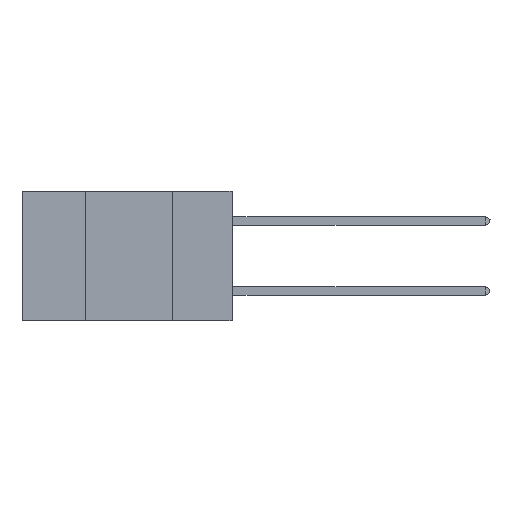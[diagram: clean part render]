
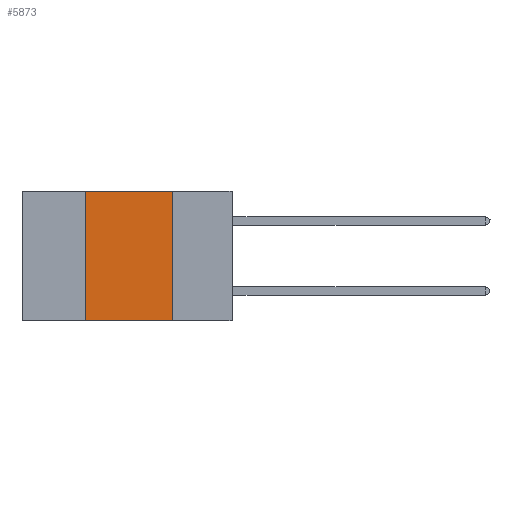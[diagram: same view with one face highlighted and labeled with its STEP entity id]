
A CAD part, left-side view. The second image highlights one B-rep face of the part: STEP entity #5873.
In plain terms, the highlighted planar face has unit normal (-1, 0, 0).
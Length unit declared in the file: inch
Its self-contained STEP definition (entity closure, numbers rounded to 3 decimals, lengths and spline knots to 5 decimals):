
#639 = VECTOR ( 'NONE', #10328, 39.37008 ) ;
#781 = VECTOR ( 'NONE', #17531, 39.37008 ) ;
#862 = EDGE_CURVE ( 'NONE', #16642, #2474, #8968, .T. ) ;
#1732 = DIRECTION ( 'NONE',  ( 1., 0., 0. ) ) ;
#2474 = VERTEX_POINT ( 'NONE', #2583 ) ;
#2583 = CARTESIAN_POINT ( 'NONE',  ( 0., 0.17, -0.37 ) ) ;
#3171 = CARTESIAN_POINT ( 'NONE',  ( 0., 0.17, 0. ) ) ;
#3392 = LINE ( 'NONE', #10825, #6792 ) ;
#3987 = AXIS2_PLACEMENT_3D ( 'NONE', #11845, #1732, #16281 ) ;
#5276 = VECTOR ( 'NONE', #15677, 39.37008 ) ;
#5873 = ADVANCED_FACE ( 'NONE', ( #15028 ), #18008, .F. ) ;
#6792 = VECTOR ( 'NONE', #7644, 39.37008 ) ;
#7164 = CARTESIAN_POINT ( 'NONE',  ( 0., 0.42, 0. ) ) ;
#7200 = LINE ( 'NONE', #14422, #5276 ) ;
#7644 = DIRECTION ( 'NONE',  ( 0., -1., 0. ) ) ;
#7986 = VERTEX_POINT ( 'NONE', #9583 ) ;
#8968 = LINE ( 'NONE', #3171, #639 ) ;
#9583 = CARTESIAN_POINT ( 'NONE',  ( 0., 0.42, -0.37 ) ) ;
#9607 = EDGE_CURVE ( 'NONE', #17743, #16642, #3392, .T. ) ;
#10127 = CARTESIAN_POINT ( 'NONE',  ( 0., 0.42, 0. ) ) ;
#10328 = DIRECTION ( 'NONE',  ( 0., 0., -1. ) ) ;
#10770 = EDGE_CURVE ( 'NONE', #7986, #2474, #7200, .T. ) ;
#10825 = CARTESIAN_POINT ( 'NONE',  ( 0., 0.6, 0. ) ) ;
#10994 = CARTESIAN_POINT ( 'NONE',  ( 0., 0.17, 0. ) ) ;
#11845 = CARTESIAN_POINT ( 'NONE',  ( 0., 0.6, 0. ) ) ;
#12865 = ORIENTED_EDGE ( 'NONE', *, *, #10770, .T. ) ;
#13045 = EDGE_LOOP ( 'NONE', ( #17592, #13326, #13464, #12865 ) ) ;
#13326 = ORIENTED_EDGE ( 'NONE', *, *, #9607, .F. ) ;
#13464 = ORIENTED_EDGE ( 'NONE', *, *, #16815, .F. ) ;
#14422 = CARTESIAN_POINT ( 'NONE',  ( 0., 0.6, -0.37 ) ) ;
#14449 = LINE ( 'NONE', #10127, #781 ) ;
#15028 = FACE_OUTER_BOUND ( 'NONE', #13045, .T. ) ;
#15677 = DIRECTION ( 'NONE',  ( 0., -1., 0. ) ) ;
#16281 = DIRECTION ( 'NONE',  ( 0., 0., -1. ) ) ;
#16642 = VERTEX_POINT ( 'NONE', #10994 ) ;
#16815 = EDGE_CURVE ( 'NONE', #7986, #17743, #14449, .T. ) ;
#17531 = DIRECTION ( 'NONE',  ( 0., 0., 1. ) ) ;
#17592 = ORIENTED_EDGE ( 'NONE', *, *, #862, .F. ) ;
#17743 = VERTEX_POINT ( 'NONE', #7164 ) ;
#18008 = PLANE ( 'NONE',  #3987 ) ;
